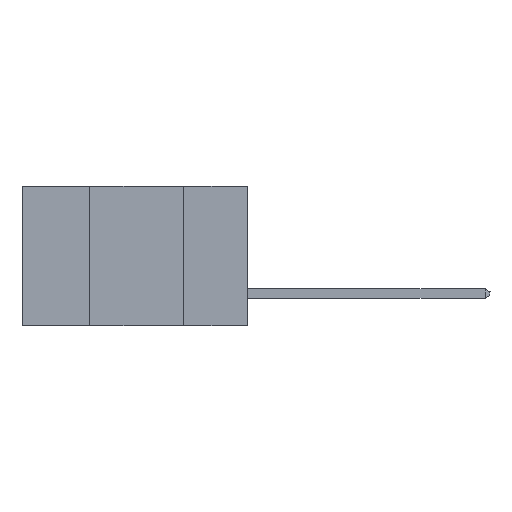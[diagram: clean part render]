
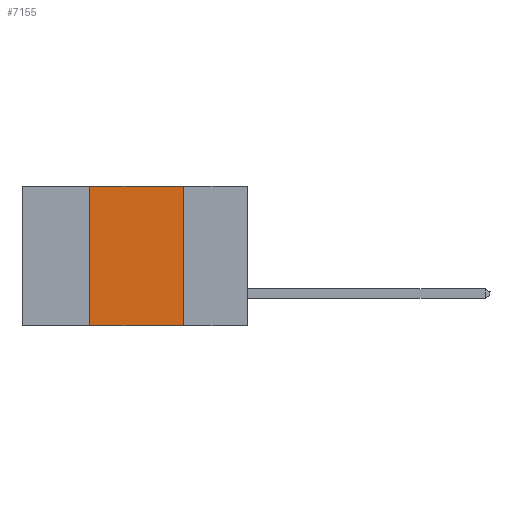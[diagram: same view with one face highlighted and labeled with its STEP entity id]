
A CAD part, left-side view. The second image highlights one B-rep face of the part: STEP entity #7155.
In plain terms, the highlighted planar face has unit normal (-1, 0, 0).
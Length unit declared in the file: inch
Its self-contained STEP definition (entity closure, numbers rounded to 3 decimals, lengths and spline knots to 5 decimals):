
#963 = CARTESIAN_POINT ( 'NONE',  ( 0., 0.17, -0.37 ) ) ;
#1143 = DIRECTION ( 'NONE',  ( 0., -1., 0. ) ) ;
#1253 = DIRECTION ( 'NONE',  ( 1., 0., 0. ) ) ;
#1523 = CARTESIAN_POINT ( 'NONE',  ( 0., 0.6, 0. ) ) ;
#2609 = VERTEX_POINT ( 'NONE', #8593 ) ;
#2902 = EDGE_LOOP ( 'NONE', ( #10625, #8474, #4371, #6166 ) ) ;
#4145 = LINE ( 'NONE', #1523, #12088 ) ;
#4371 = ORIENTED_EDGE ( 'NONE', *, *, #10241, .F. ) ;
#4413 = CARTESIAN_POINT ( 'NONE',  ( 0., 0.17, -0.37 ) ) ;
#5796 = LINE ( 'NONE', #7456, #7499 ) ;
#5983 = EDGE_CURVE ( 'NONE', #2609, #9969, #4145, .T. ) ;
#6166 = ORIENTED_EDGE ( 'NONE', *, *, #15487, .T. ) ;
#6314 = LINE ( 'NONE', #6698, #12929 ) ;
#6380 = VERTEX_POINT ( 'NONE', #4413 ) ;
#6591 = EDGE_CURVE ( 'NONE', #9969, #6380, #7074, .T. ) ;
#6698 = CARTESIAN_POINT ( 'NONE',  ( 0., 0.6, -0.37 ) ) ;
#6760 = CARTESIAN_POINT ( 'NONE',  ( 0., 0.42, -0.37 ) ) ;
#7074 = LINE ( 'NONE', #963, #13638 ) ;
#7155 = ADVANCED_FACE ( 'NONE', ( #13819 ), #13616, .F. ) ;
#7456 = CARTESIAN_POINT ( 'NONE',  ( 0., 0.42, -0.37 ) ) ;
#7499 = VECTOR ( 'NONE', #13805, 39.37008 ) ;
#8474 = ORIENTED_EDGE ( 'NONE', *, *, #5983, .F. ) ;
#8593 = CARTESIAN_POINT ( 'NONE',  ( 0., 0.42, 0. ) ) ;
#9422 = CARTESIAN_POINT ( 'NONE',  ( 0., 0.17, 0. ) ) ;
#9969 = VERTEX_POINT ( 'NONE', #9422 ) ;
#10241 = EDGE_CURVE ( 'NONE', #17648, #2609, #5796, .T. ) ;
#10625 = ORIENTED_EDGE ( 'NONE', *, *, #6591, .F. ) ;
#12088 = VECTOR ( 'NONE', #1143, 39.37008 ) ;
#12929 = VECTOR ( 'NONE', #19278, 39.37008 ) ;
#13616 = PLANE ( 'NONE',  #17819 ) ;
#13638 = VECTOR ( 'NONE', #16531, 39.37008 ) ;
#13805 = DIRECTION ( 'NONE',  ( 0., 0., 1. ) ) ;
#13819 = FACE_OUTER_BOUND ( 'NONE', #2902, .T. ) ;
#15178 = DIRECTION ( 'NONE',  ( 0., 0., -1. ) ) ;
#15392 = CARTESIAN_POINT ( 'NONE',  ( 0., 0.6, 0. ) ) ;
#15487 = EDGE_CURVE ( 'NONE', #17648, #6380, #6314, .T. ) ;
#16531 = DIRECTION ( 'NONE',  ( 0., 0., -1. ) ) ;
#17648 = VERTEX_POINT ( 'NONE', #6760 ) ;
#17819 = AXIS2_PLACEMENT_3D ( 'NONE', #15392, #1253, #15178 ) ;
#19278 = DIRECTION ( 'NONE',  ( 0., -1., 0. ) ) ;
